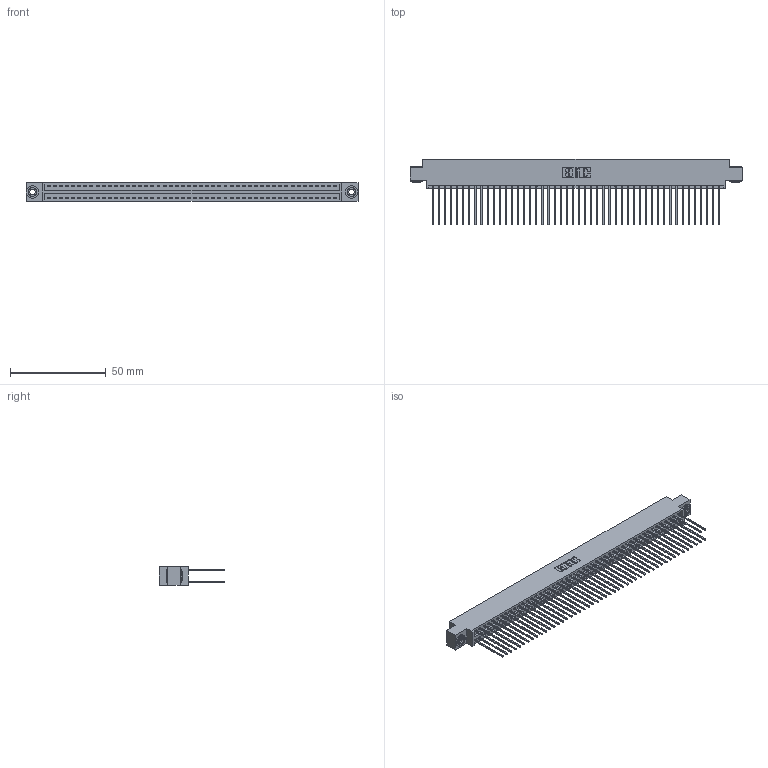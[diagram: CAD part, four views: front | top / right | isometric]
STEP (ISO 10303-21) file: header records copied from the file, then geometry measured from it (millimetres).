
FILE_DESCRIPTION (( 'STEP AP203' ), '1' );
FILE_NAME ('396-096-541-803.STEP', '2019-11-02T16:44:36', ( '' ), ( '' ), 'SwSTEP 2.0', 'SolidWorks 2016', '' );
FILE_SCHEMA (( 'CONFIG_CONTROL_DESIGN' ));
Length unit declared in the file: inch
Products named in the file (4): 346 Part_0.170 Offset - 0.156 Dia-TH; 345-292-001_345-293-141; 345-250-002_345-250-002-102; 396-096-541-803
Assembly tree (99 placements, depth 2):
  396-096-541-803
    346 Part_0.170 Offset - 0.156 Dia-TH
    345-292-001_345-293-141  x96
    345-250-002_345-250-002-102  x2
Bounding box: 172.97 x 34.29 x 9.4 mm (x, y, z)
Volume: 17329.2 mm3; surface area: 26949.7 mm2
Topology: 99 solids, 99 shells, 5156 faces, 15297 edges, 10066 vertices
Faces by surface type: plane 3450, cylinder 1698, cone 8
Entity records: 31318 total; most frequent: CARTESIAN_POINT 5131, ORIENTED_EDGE 5058, DIRECTION 4603, EDGE_CURVE 2529, VECTOR 2181, LINE 2181, VERTEX_POINT 1682, AXIS2_PLACEMENT_3D 1211
